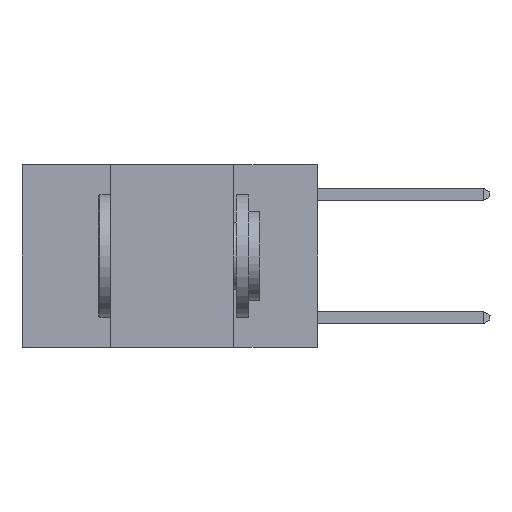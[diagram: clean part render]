
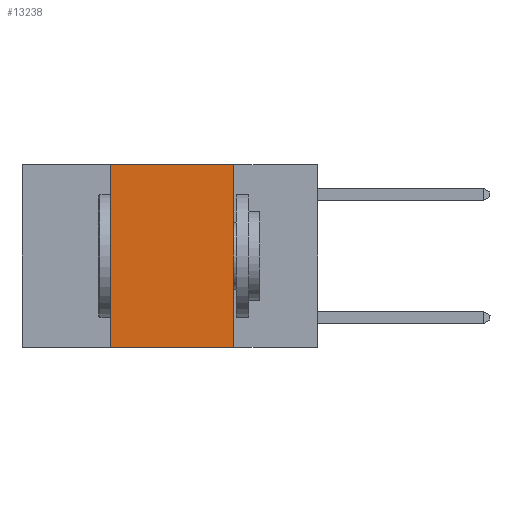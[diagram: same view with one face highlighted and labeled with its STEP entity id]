
A CAD part, left-side view. The second image highlights one B-rep face of the part: STEP entity #13238.
In plain terms, the highlighted planar face has unit normal (-1, 0, 0).
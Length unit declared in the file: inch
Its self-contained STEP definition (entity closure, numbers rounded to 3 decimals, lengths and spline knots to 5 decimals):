
#367 = DIRECTION ( 'NONE',  ( 0., 0., 1. ) ) ;
#1179 = CARTESIAN_POINT ( 'NONE',  ( 0., 0.42, -0.37 ) ) ;
#1404 = VERTEX_POINT ( 'NONE', #20878 ) ;
#1914 = DIRECTION ( 'NONE',  ( 0., -1., 0. ) ) ;
#2010 = ORIENTED_EDGE ( 'NONE', *, *, #8318, .F. ) ;
#3760 = ORIENTED_EDGE ( 'NONE', *, *, #19153, .T. ) ;
#3851 = CARTESIAN_POINT ( 'NONE',  ( 0., 0.6, -0.37 ) ) ;
#5421 = EDGE_CURVE ( 'NONE', #22168, #1404, #7769, .T. ) ;
#5719 = VERTEX_POINT ( 'NONE', #1179 ) ;
#5776 = DIRECTION ( 'NONE',  ( 0., 0., -1. ) ) ;
#5787 = DIRECTION ( 'NONE',  ( 0., -1., 0. ) ) ;
#6595 = AXIS2_PLACEMENT_3D ( 'NONE', #19288, #10341, #22849 ) ;
#7133 = EDGE_LOOP ( 'NONE', ( #2010, #7656, #22527, #3760 ) ) ;
#7656 = ORIENTED_EDGE ( 'NONE', *, *, #5421, .F. ) ;
#7769 = LINE ( 'NONE', #18340, #17349 ) ;
#8318 = EDGE_CURVE ( 'NONE', #1404, #17519, #11171, .T. ) ;
#10341 = DIRECTION ( 'NONE',  ( 1., 0., 0. ) ) ;
#11171 = LINE ( 'NONE', #18467, #11719 ) ;
#11466 = CARTESIAN_POINT ( 'NONE',  ( 0., 0.42, 0. ) ) ;
#11719 = VECTOR ( 'NONE', #5776, 39.37008 ) ;
#12067 = VECTOR ( 'NONE', #367, 39.37008 ) ;
#13238 = ADVANCED_FACE ( 'NONE', ( #21118 ), #21094, .F. ) ;
#14326 = EDGE_CURVE ( 'NONE', #5719, #22168, #16286, .T. ) ;
#15600 = CARTESIAN_POINT ( 'NONE',  ( 0., 0.17, -0.37 ) ) ;
#16132 = VECTOR ( 'NONE', #5787, 39.37008 ) ;
#16286 = LINE ( 'NONE', #11466, #12067 ) ;
#16691 = LINE ( 'NONE', #3851, #16132 ) ;
#17349 = VECTOR ( 'NONE', #1914, 39.37008 ) ;
#17519 = VERTEX_POINT ( 'NONE', #15600 ) ;
#17753 = CARTESIAN_POINT ( 'NONE',  ( 0., 0.42, 0. ) ) ;
#18340 = CARTESIAN_POINT ( 'NONE',  ( 0., 0.6, 0. ) ) ;
#18467 = CARTESIAN_POINT ( 'NONE',  ( 0., 0.17, 0. ) ) ;
#19153 = EDGE_CURVE ( 'NONE', #5719, #17519, #16691, .T. ) ;
#19288 = CARTESIAN_POINT ( 'NONE',  ( 0., 0.6, 0. ) ) ;
#20878 = CARTESIAN_POINT ( 'NONE',  ( 0., 0.17, 0. ) ) ;
#21094 = PLANE ( 'NONE',  #6595 ) ;
#21118 = FACE_OUTER_BOUND ( 'NONE', #7133, .T. ) ;
#22168 = VERTEX_POINT ( 'NONE', #17753 ) ;
#22527 = ORIENTED_EDGE ( 'NONE', *, *, #14326, .F. ) ;
#22849 = DIRECTION ( 'NONE',  ( 0., 0., -1. ) ) ;
